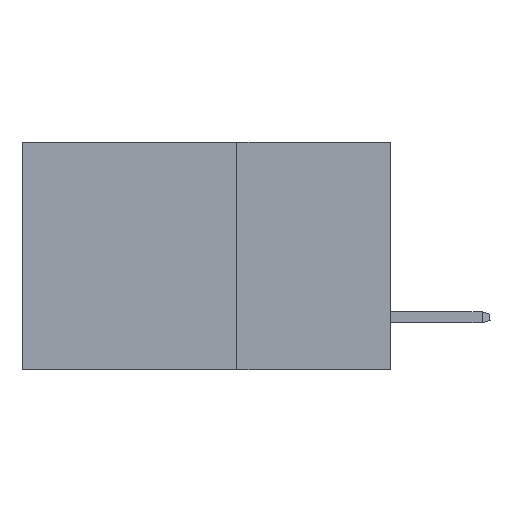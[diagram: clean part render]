
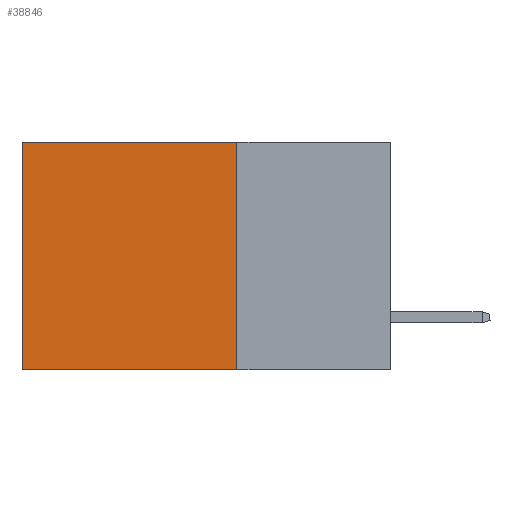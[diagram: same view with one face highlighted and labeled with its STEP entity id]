
A CAD part, left-side view. The second image highlights one B-rep face of the part: STEP entity #38846.
In plain terms, the highlighted planar face has unit normal (-1, 0, 0).
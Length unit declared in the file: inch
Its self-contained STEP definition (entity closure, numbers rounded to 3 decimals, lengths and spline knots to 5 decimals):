
#2284 = VECTOR ( 'NONE', #45315, 39.37008 ) ;
#3620 = VERTEX_POINT ( 'NONE', #11461 ) ;
#3847 = DIRECTION ( 'NONE',  ( 0., 0., -1. ) ) ;
#4330 = ORIENTED_EDGE ( 'NONE', *, *, #34007, .T. ) ;
#4933 = ORIENTED_EDGE ( 'NONE', *, *, #10771, .F. ) ;
#5044 = VERTEX_POINT ( 'NONE', #44188 ) ;
#6495 = DIRECTION ( 'NONE',  ( 0., 0., -1. ) ) ;
#10771 = EDGE_CURVE ( 'NONE', #12122, #5044, #47027, .T. ) ;
#11461 = CARTESIAN_POINT ( 'NONE',  ( 0.2875, 0.6, 0. ) ) ;
#12056 = DIRECTION ( 'NONE',  ( 0., 0., -1. ) ) ;
#12122 = VERTEX_POINT ( 'NONE', #16484 ) ;
#12350 = VECTOR ( 'NONE', #40695, 39.37008 ) ;
#12467 = FACE_OUTER_BOUND ( 'NONE', #35186, .T. ) ;
#13911 = CARTESIAN_POINT ( 'NONE',  ( 0.2875, 0.25, 0. ) ) ;
#16484 = CARTESIAN_POINT ( 'NONE',  ( 0.2875, 0.25, 0. ) ) ;
#19567 = CARTESIAN_POINT ( 'NONE',  ( 0.2875, 0.6, 0. ) ) ;
#22845 = CARTESIAN_POINT ( 'NONE',  ( 0.2875, 0.25, -0.37 ) ) ;
#23654 = VECTOR ( 'NONE', #6495, 39.37008 ) ;
#26379 = DIRECTION ( 'NONE',  ( 1., 0., 0. ) ) ;
#28367 = EDGE_CURVE ( 'NONE', #5044, #45621, #35156, .T. ) ;
#29323 = CARTESIAN_POINT ( 'NONE',  ( 0.2875, 0.25, 0. ) ) ;
#31285 = AXIS2_PLACEMENT_3D ( 'NONE', #37772, #26379, #3847 ) ;
#34007 = EDGE_CURVE ( 'NONE', #12122, #3620, #44130, .T. ) ;
#35156 = LINE ( 'NONE', #22845, #2284 ) ;
#35186 = EDGE_LOOP ( 'NONE', ( #46788, #38065, #4933, #4330 ) ) ;
#35838 = LINE ( 'NONE', #19567, #44310 ) ;
#37772 = CARTESIAN_POINT ( 'NONE',  ( 0.2875, 0.25, 0. ) ) ;
#38065 = ORIENTED_EDGE ( 'NONE', *, *, #28367, .F. ) ;
#38379 = EDGE_CURVE ( 'NONE', #3620, #45621, #35838, .T. ) ;
#38846 = ADVANCED_FACE ( 'NONE', ( #12467 ), #49573, .F. ) ;
#40695 = DIRECTION ( 'NONE',  ( 0., 1., 0. ) ) ;
#43760 = CARTESIAN_POINT ( 'NONE',  ( 0.2875, 0.6, -0.37 ) ) ;
#44130 = LINE ( 'NONE', #13911, #12350 ) ;
#44188 = CARTESIAN_POINT ( 'NONE',  ( 0.2875, 0.25, -0.37 ) ) ;
#44310 = VECTOR ( 'NONE', #12056, 39.37008 ) ;
#45315 = DIRECTION ( 'NONE',  ( 0., 1., 0. ) ) ;
#45621 = VERTEX_POINT ( 'NONE', #43760 ) ;
#46788 = ORIENTED_EDGE ( 'NONE', *, *, #38379, .T. ) ;
#47027 = LINE ( 'NONE', #29323, #23654 ) ;
#49573 = PLANE ( 'NONE',  #31285 ) ;
